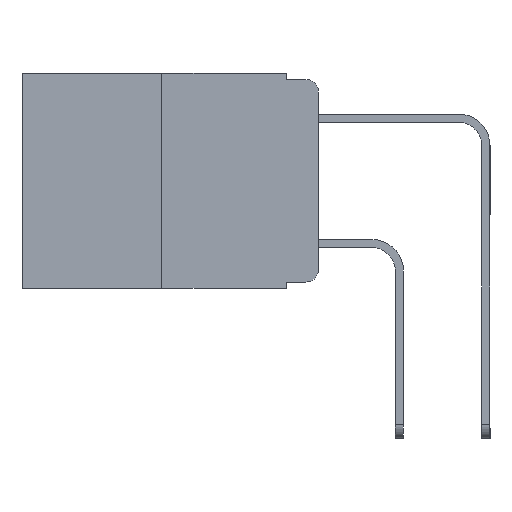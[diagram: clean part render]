
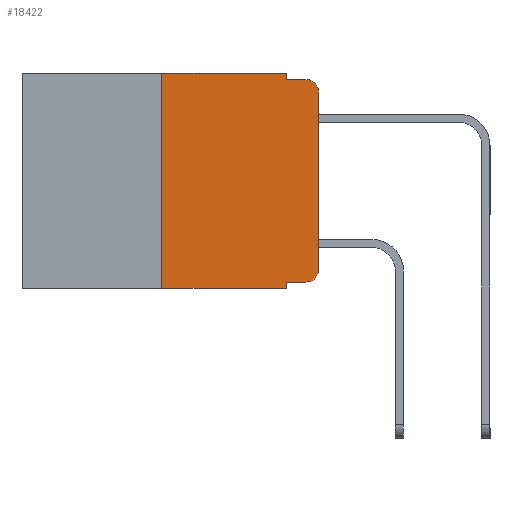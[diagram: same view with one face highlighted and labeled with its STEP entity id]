
A CAD part, left-side view. The second image highlights one B-rep face of the part: STEP entity #18422.
In plain terms, the highlighted planar face has unit normal (-1, 0, 0).
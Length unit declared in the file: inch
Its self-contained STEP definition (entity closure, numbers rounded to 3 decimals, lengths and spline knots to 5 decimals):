
#468 = LINE ( 'NONE', #8247, #9877 ) ;
#513 = VECTOR ( 'NONE', #3557, 39.37008 ) ;
#1187 = CARTESIAN_POINT ( 'NONE',  ( 0., 0., -0.313 ) ) ;
#1336 = EDGE_CURVE ( 'NONE', #9467, #7805, #16379, .T. ) ;
#1914 = DIRECTION ( 'NONE',  ( 0., -1., 0. ) ) ;
#1998 = ORIENTED_EDGE ( 'NONE', *, *, #1336, .F. ) ;
#2266 = ORIENTED_EDGE ( 'NONE', *, *, #19208, .F. ) ;
#2502 = LINE ( 'NONE', #15701, #11883 ) ;
#2634 = CARTESIAN_POINT ( 'NONE',  ( 0., 0.473, 0. ) ) ;
#2701 = DIRECTION ( 'NONE',  ( 0., -1., 0. ) ) ;
#3136 = EDGE_CURVE ( 'NONE', #19494, #7805, #7362, .T. ) ;
#3422 = CARTESIAN_POINT ( 'NONE',  ( 0., 0.051, 0. ) ) ;
#3557 = DIRECTION ( 'NONE',  ( 0., -1., 0. ) ) ;
#3864 = LINE ( 'NONE', #10130, #8276 ) ;
#3984 = VERTEX_POINT ( 'NONE', #7083 ) ;
#4140 = CARTESIAN_POINT ( 'NONE',  ( 0., 0.02, -0.01 ) ) ;
#4164 = EDGE_CURVE ( 'NONE', #8874, #7416, #5527, .T. ) ;
#4369 = ORIENTED_EDGE ( 'NONE', *, *, #13391, .T. ) ;
#4561 = DIRECTION ( 'NONE',  ( 0., 0., 1. ) ) ;
#4802 = EDGE_CURVE ( 'NONE', #7416, #3984, #7577, .T. ) ;
#5527 = LINE ( 'NONE', #2634, #513 ) ;
#5681 = CARTESIAN_POINT ( 'NONE',  ( 0., 0.051, -0.01 ) ) ;
#5809 = ORIENTED_EDGE ( 'NONE', *, *, #10132, .F. ) ;
#5876 = VERTEX_POINT ( 'NONE', #11138 ) ;
#6098 = ORIENTED_EDGE ( 'NONE', *, *, #22898, .T. ) ;
#6159 = DIRECTION ( 'NONE',  ( -1., 0., 0. ) ) ;
#7047 = AXIS2_PLACEMENT_3D ( 'NONE', #9871, #22575, #11736 ) ;
#7083 = CARTESIAN_POINT ( 'NONE',  ( 0., 0.051, -0.01 ) ) ;
#7103 = VECTOR ( 'NONE', #1914, 39.37008 ) ;
#7362 = LINE ( 'NONE', #8929, #16620 ) ;
#7416 = VERTEX_POINT ( 'NONE', #19132 ) ;
#7492 = EDGE_LOOP ( 'NONE', ( #6098, #21338, #2266, #7885, #23526, #5809, #10773, #1998, #13109, #4369 ) ) ;
#7510 = EDGE_CURVE ( 'NONE', #9467, #5876, #3864, .T. ) ;
#7577 = LINE ( 'NONE', #23584, #11921 ) ;
#7613 = VERTEX_POINT ( 'NONE', #1187 ) ;
#7805 = VERTEX_POINT ( 'NONE', #23822 ) ;
#7885 = ORIENTED_EDGE ( 'NONE', *, *, #4802, .F. ) ;
#8247 = CARTESIAN_POINT ( 'NONE',  ( 0., 0.25, 0. ) ) ;
#8276 = VECTOR ( 'NONE', #22913, 39.37008 ) ;
#8874 = VERTEX_POINT ( 'NONE', #15576 ) ;
#8929 = CARTESIAN_POINT ( 'NONE',  ( 0., 0.473, -0.343 ) ) ;
#9467 = VERTEX_POINT ( 'NONE', #13760 ) ;
#9871 = CARTESIAN_POINT ( 'NONE',  ( 0., 0.02, -0.313 ) ) ;
#9877 = VECTOR ( 'NONE', #21064, 39.37008 ) ;
#10130 = CARTESIAN_POINT ( 'NONE',  ( 0., 0.051, -0.333 ) ) ;
#10132 = EDGE_CURVE ( 'NONE', #19494, #8874, #468, .T. ) ;
#10175 = CARTESIAN_POINT ( 'NONE',  ( 0., 0.25, -0.343 ) ) ;
#10710 = DIRECTION ( 'NONE',  ( 0., 0., -1. ) ) ;
#10773 = ORIENTED_EDGE ( 'NONE', *, *, #3136, .T. ) ;
#11085 = CIRCLE ( 'NONE', #7047, 0.02 ) ;
#11138 = CARTESIAN_POINT ( 'NONE',  ( 0., 0.02, -0.333 ) ) ;
#11736 = DIRECTION ( 'NONE',  ( 0., 0., -1. ) ) ;
#11883 = VECTOR ( 'NONE', #4561, 39.37008 ) ;
#11921 = VECTOR ( 'NONE', #23632, 39.37008 ) ;
#13109 = ORIENTED_EDGE ( 'NONE', *, *, #7510, .T. ) ;
#13391 = EDGE_CURVE ( 'NONE', #5876, #7613, #11085, .T. ) ;
#13472 = CIRCLE ( 'NONE', #15015, 0.02 ) ;
#13494 = DIRECTION ( 'NONE',  ( 0., 0., -1. ) ) ;
#13760 = CARTESIAN_POINT ( 'NONE',  ( 0., 0.051, -0.333 ) ) ;
#13957 = VERTEX_POINT ( 'NONE', #4140 ) ;
#14351 = PLANE ( 'NONE',  #18251 ) ;
#14929 = VERTEX_POINT ( 'NONE', #21723 ) ;
#15015 = AXIS2_PLACEMENT_3D ( 'NONE', #17248, #6159, #19076 ) ;
#15576 = CARTESIAN_POINT ( 'NONE',  ( 0., 0.25, 0. ) ) ;
#15701 = CARTESIAN_POINT ( 'NONE',  ( 0., 0., 0. ) ) ;
#16379 = LINE ( 'NONE', #3422, #20626 ) ;
#16620 = VECTOR ( 'NONE', #2701, 39.37008 ) ;
#16927 = FACE_OUTER_BOUND ( 'NONE', #7492, .T. ) ;
#16939 = LINE ( 'NONE', #5681, #7103 ) ;
#17248 = CARTESIAN_POINT ( 'NONE',  ( 0., 0.02, -0.03 ) ) ;
#18037 = CARTESIAN_POINT ( 'NONE',  ( 0., 0.473, 0. ) ) ;
#18151 = EDGE_CURVE ( 'NONE', #14929, #13957, #13472, .T. ) ;
#18251 = AXIS2_PLACEMENT_3D ( 'NONE', #18037, #21630, #10710 ) ;
#18422 = ADVANCED_FACE ( 'NONE', ( #16927 ), #14351, .F. ) ;
#19076 = DIRECTION ( 'NONE',  ( 0., 0., -1. ) ) ;
#19132 = CARTESIAN_POINT ( 'NONE',  ( 0., 0.051, 0. ) ) ;
#19208 = EDGE_CURVE ( 'NONE', #3984, #13957, #16939, .T. ) ;
#19494 = VERTEX_POINT ( 'NONE', #10175 ) ;
#20626 = VECTOR ( 'NONE', #13494, 39.37008 ) ;
#21064 = DIRECTION ( 'NONE',  ( 0., 0., 1. ) ) ;
#21338 = ORIENTED_EDGE ( 'NONE', *, *, #18151, .T. ) ;
#21630 = DIRECTION ( 'NONE',  ( 1., 0., 0. ) ) ;
#21723 = CARTESIAN_POINT ( 'NONE',  ( 0., 0., -0.03 ) ) ;
#22575 = DIRECTION ( 'NONE',  ( -1., 0., 0. ) ) ;
#22898 = EDGE_CURVE ( 'NONE', #7613, #14929, #2502, .T. ) ;
#22913 = DIRECTION ( 'NONE',  ( 0., -1., 0. ) ) ;
#23526 = ORIENTED_EDGE ( 'NONE', *, *, #4164, .F. ) ;
#23584 = CARTESIAN_POINT ( 'NONE',  ( 0., 0.051, 0. ) ) ;
#23632 = DIRECTION ( 'NONE',  ( 0., 0., -1. ) ) ;
#23822 = CARTESIAN_POINT ( 'NONE',  ( 0., 0.051, -0.343 ) ) ;
